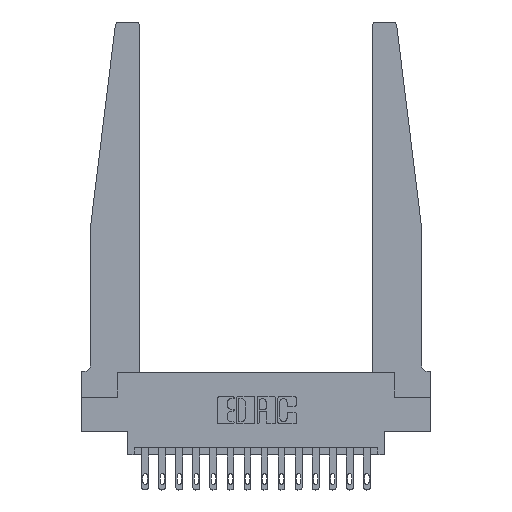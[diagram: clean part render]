
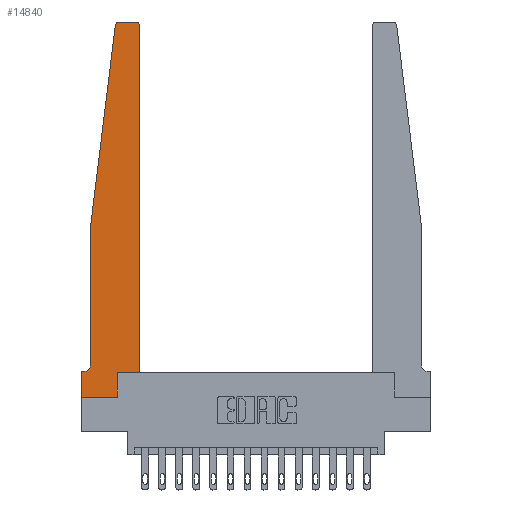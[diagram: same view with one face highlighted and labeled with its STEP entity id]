
A CAD part, top view. The second image highlights one B-rep face of the part: STEP entity #14840.
In plain terms, the highlighted planar face has unit normal (0, 0, 1).
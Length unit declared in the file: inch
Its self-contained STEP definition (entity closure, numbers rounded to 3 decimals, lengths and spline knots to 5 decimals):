
#243 = CARTESIAN_POINT ( 'NONE',  ( 0., 0.1875, 0.37 ) ) ;
#485 = ORIENTED_EDGE ( 'NONE', *, *, #13314, .T. ) ;
#619 = CARTESIAN_POINT ( 'NONE',  ( 0., 0., 0.37 ) ) ;
#879 = DIRECTION ( 'NONE',  ( 1., 0., 0. ) ) ;
#1126 = LINE ( 'NONE', #3973, #2273 ) ;
#1275 = CARTESIAN_POINT ( 'NONE',  ( 0.015, 0.1875, 0.37 ) ) ;
#1286 = DIRECTION ( 'NONE',  ( -1., 0., 0. ) ) ;
#1669 = EDGE_CURVE ( 'NONE', #5522, #17490, #8532, .T. ) ;
#1777 = CIRCLE ( 'NONE', #12062, 0.03 ) ;
#2017 = ORIENTED_EDGE ( 'NONE', *, *, #17882, .T. ) ;
#2273 = VECTOR ( 'NONE', #8127, 39.37008 ) ;
#2387 = VECTOR ( 'NONE', #8461, 39.37008 ) ;
#2474 = ORIENTED_EDGE ( 'NONE', *, *, #9259, .T. ) ;
#2557 = DIRECTION ( 'NONE',  ( 1., 0., 0. ) ) ;
#2787 = CARTESIAN_POINT ( 'NONE',  ( 0.065, 1.25, 0.37 ) ) ;
#2791 = EDGE_CURVE ( 'NONE', #11241, #14777, #18102, .T. ) ;
#2814 = DIRECTION ( 'NONE',  ( 0., 0., 1. ) ) ;
#2851 = VERTEX_POINT ( 'NONE', #1275 ) ;
#3035 = VERTEX_POINT ( 'NONE', #13227 ) ;
#3329 = DIRECTION ( 'NONE',  ( 1., 0., 0. ) ) ;
#3734 = EDGE_CURVE ( 'NONE', #17490, #4630, #1777, .T. ) ;
#3973 = CARTESIAN_POINT ( 'NONE',  ( 0., 0., 0.37 ) ) ;
#4168 = DIRECTION ( 'NONE',  ( 0., 0., 1. ) ) ;
#4520 = DIRECTION ( 'NONE',  ( 1., 0., 0. ) ) ;
#4526 = DIRECTION ( 'NONE',  ( 0., 1., 0. ) ) ;
#4630 = VERTEX_POINT ( 'NONE', #5418 ) ;
#5029 = VECTOR ( 'NONE', #3329, 39.37008 ) ;
#5042 = EDGE_CURVE ( 'NONE', #16438, #3035, #10171, .T. ) ;
#5228 = CARTESIAN_POINT ( 'NONE',  ( 0.27653, 2.75, 0.37 ) ) ;
#5418 = CARTESIAN_POINT ( 'NONE',  ( 0.24675, 2.72367, 0.37 ) ) ;
#5522 = VERTEX_POINT ( 'NONE', #14107 ) ;
#5653 = ORIENTED_EDGE ( 'NONE', *, *, #2791, .T. ) ;
#5881 = LINE ( 'NONE', #11506, #2387 ) ;
#6012 = DIRECTION ( 'NONE',  ( 0., 0., -1. ) ) ;
#6252 = ORIENTED_EDGE ( 'NONE', *, *, #1669, .T. ) ;
#6398 = LINE ( 'NONE', #7517, #12394 ) ;
#6405 = CARTESIAN_POINT ( 'NONE',  ( 0.395, 2.72, 0.37 ) ) ;
#6431 = VERTEX_POINT ( 'NONE', #15343 ) ;
#6707 = ORIENTED_EDGE ( 'NONE', *, *, #7949, .T. ) ;
#6811 = CARTESIAN_POINT ( 'NONE',  ( 0.065, 0.1875, 0.37 ) ) ;
#7125 = CARTESIAN_POINT ( 'NONE',  ( 0.425, 0.18, 0.37 ) ) ;
#7165 = CIRCLE ( 'NONE', #10718, 0.03 ) ;
#7328 = CARTESIAN_POINT ( 'NONE',  ( 0.065, 0.2375, 0.37 ) ) ;
#7517 = CARTESIAN_POINT ( 'NONE',  ( 0.065, 1.25, 0.37 ) ) ;
#7878 = DIRECTION ( 'NONE',  ( 0., 0., 1. ) ) ;
#7949 = EDGE_CURVE ( 'NONE', #6431, #12790, #12385, .T. ) ;
#8127 = DIRECTION ( 'NONE',  ( 0., -1., 0. ) ) ;
#8167 = CARTESIAN_POINT ( 'NONE',  ( 0.2605, 0.18, 0.37 ) ) ;
#8261 = AXIS2_PLACEMENT_3D ( 'NONE', #13298, #6012, #11828 ) ;
#8461 = DIRECTION ( 'NONE',  ( 0., 1., 0. ) ) ;
#8532 = LINE ( 'NONE', #15619, #9335 ) ;
#8671 = CARTESIAN_POINT ( 'NONE',  ( 0.27653, 2.72, 0.37 ) ) ;
#9020 = VECTOR ( 'NONE', #14129, 39.37008 ) ;
#9251 = ORIENTED_EDGE ( 'NONE', *, *, #15070, .T. ) ;
#9259 = EDGE_CURVE ( 'NONE', #11447, #11241, #1126, .T. ) ;
#9298 = LINE ( 'NONE', #6811, #17876 ) ;
#9335 = VECTOR ( 'NONE', #12951, 39.37008 ) ;
#9454 = CARTESIAN_POINT ( 'NONE',  ( 0., 0.1875, 0.37 ) ) ;
#9621 = EDGE_CURVE ( 'NONE', #2851, #11447, #9298, .T. ) ;
#10171 = LINE ( 'NONE', #7125, #13715 ) ;
#10447 = CARTESIAN_POINT ( 'NONE',  ( 0.425, 0.18, 0.37 ) ) ;
#10718 = AXIS2_PLACEMENT_3D ( 'NONE', #6405, #7878, #879 ) ;
#10959 = CARTESIAN_POINT ( 'NONE',  ( 0.425, 0.18, 0.37 ) ) ;
#11070 = EDGE_LOOP ( 'NONE', ( #6252, #17578, #9251, #6707, #17794, #13211, #2474, #5653, #485, #14668, #11249, #2017 ) ) ;
#11241 = VERTEX_POINT ( 'NONE', #619 ) ;
#11249 = ORIENTED_EDGE ( 'NONE', *, *, #5042, .T. ) ;
#11447 = VERTEX_POINT ( 'NONE', #9454 ) ;
#11506 = CARTESIAN_POINT ( 'NONE',  ( 0.2605, 0.18, 0.37 ) ) ;
#11828 = DIRECTION ( 'NONE',  ( -1., 0., 0. ) ) ;
#12009 = DIRECTION ( 'NONE',  ( -0.122, -0.992, 0. ) ) ;
#12062 = AXIS2_PLACEMENT_3D ( 'NONE', #8671, #4168, #4520 ) ;
#12217 = CARTESIAN_POINT ( 'NONE',  ( 0.2605, 0., 0.37 ) ) ;
#12385 = LINE ( 'NONE', #2787, #9020 ) ;
#12394 = VECTOR ( 'NONE', #12009, 39.37008 ) ;
#12790 = VERTEX_POINT ( 'NONE', #7328 ) ;
#12855 = DIRECTION ( 'NONE',  ( 1., 0., 0. ) ) ;
#12951 = DIRECTION ( 'NONE',  ( -1., 0., 0. ) ) ;
#13211 = ORIENTED_EDGE ( 'NONE', *, *, #9621, .T. ) ;
#13227 = CARTESIAN_POINT ( 'NONE',  ( 0.425, 2.72, 0.37 ) ) ;
#13298 = CARTESIAN_POINT ( 'NONE',  ( 0.015, 0.2375, 0.37 ) ) ;
#13314 = EDGE_CURVE ( 'NONE', #14777, #18130, #5881, .T. ) ;
#13715 = VECTOR ( 'NONE', #4526, 39.37008 ) ;
#14107 = CARTESIAN_POINT ( 'NONE',  ( 0.395, 2.75, 0.37 ) ) ;
#14129 = DIRECTION ( 'NONE',  ( 0., -1., 0. ) ) ;
#14241 = EDGE_CURVE ( 'NONE', #12790, #2851, #14416, .T. ) ;
#14416 = CIRCLE ( 'NONE', #8261, 0.05 ) ;
#14668 = ORIENTED_EDGE ( 'NONE', *, *, #15401, .T. ) ;
#14777 = VERTEX_POINT ( 'NONE', #12217 ) ;
#14840 = ADVANCED_FACE ( 'NONE', ( #16997 ), #15531, .T. ) ;
#15070 = EDGE_CURVE ( 'NONE', #4630, #6431, #6398, .T. ) ;
#15343 = CARTESIAN_POINT ( 'NONE',  ( 0.065, 1.25, 0.37 ) ) ;
#15401 = EDGE_CURVE ( 'NONE', #18130, #16438, #15962, .T. ) ;
#15531 = PLANE ( 'NONE',  #16512 ) ;
#15619 = CARTESIAN_POINT ( 'NONE',  ( 0.25, 2.75, 0.37 ) ) ;
#15962 = LINE ( 'NONE', #10447, #5029 ) ;
#16373 = CARTESIAN_POINT ( 'NONE',  ( 0., 0., 0.37 ) ) ;
#16438 = VERTEX_POINT ( 'NONE', #10959 ) ;
#16512 = AXIS2_PLACEMENT_3D ( 'NONE', #243, #2814, #12855 ) ;
#16997 = FACE_OUTER_BOUND ( 'NONE', #11070, .T. ) ;
#17108 = VECTOR ( 'NONE', #2557, 39.37008 ) ;
#17490 = VERTEX_POINT ( 'NONE', #5228 ) ;
#17578 = ORIENTED_EDGE ( 'NONE', *, *, #3734, .T. ) ;
#17794 = ORIENTED_EDGE ( 'NONE', *, *, #14241, .T. ) ;
#17876 = VECTOR ( 'NONE', #1286, 39.37008 ) ;
#17882 = EDGE_CURVE ( 'NONE', #3035, #5522, #7165, .T. ) ;
#18102 = LINE ( 'NONE', #16373, #17108 ) ;
#18130 = VERTEX_POINT ( 'NONE', #8167 ) ;
